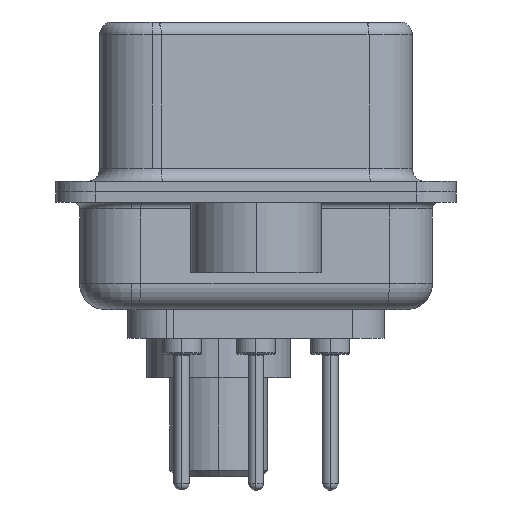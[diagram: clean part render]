
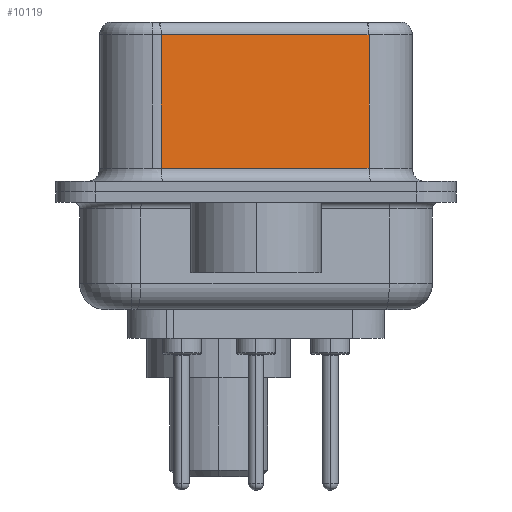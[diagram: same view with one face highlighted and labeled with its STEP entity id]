
A CAD part, left-side view. The second image highlights one B-rep face of the part: STEP entity #10119.
In plain terms, the highlighted planar face has unit normal (-0.985, -0.174, 0).
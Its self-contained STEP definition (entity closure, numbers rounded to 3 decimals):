
#584 = LINE ( 'NONE', #12378, #19956 ) ;
#1120 = CARTESIAN_POINT ( 'NONE',  ( 5.132, -4.322, 6.52 ) ) ;
#1971 = VECTOR ( 'NONE', #28779, 1000. ) ;
#3757 = VERTEX_POINT ( 'NONE', #9534 ) ;
#4213 = EDGE_LOOP ( 'NONE', ( #10689, #11433, #23676, #14604 ) ) ;
#5668 = DIRECTION ( 'NONE',  ( 0., 0., -1. ) ) ;
#5720 = PLANE ( 'NONE',  #8246 ) ;
#8246 = AXIS2_PLACEMENT_3D ( 'NONE', #1120, #19290, #12423 ) ;
#8667 = LINE ( 'NONE', #21960, #9747 ) ;
#9534 = CARTESIAN_POINT ( 'NONE',  ( 5.132, -4.322, 6.02 ) ) ;
#9747 = VECTOR ( 'NONE', #5668, 1000. ) ;
#9771 = VERTEX_POINT ( 'NONE', #20661 ) ;
#10119 = ADVANCED_FACE ( 'NONE', ( #22424 ), #5720, .F. ) ;
#10689 = ORIENTED_EDGE ( 'NONE', *, *, #27146, .F. ) ;
#11310 = VERTEX_POINT ( 'NONE', #18803 ) ;
#11433 = ORIENTED_EDGE ( 'NONE', *, *, #15634, .T. ) ;
#12378 = CARTESIAN_POINT ( 'NONE',  ( 5.132, -4.322, 0.9 ) ) ;
#12384 = LINE ( 'NONE', #28675, #1971 ) ;
#12423 = DIRECTION ( 'NONE',  ( -0.174, 0.985, 0. ) ) ;
#13137 = LINE ( 'NONE', #22871, #29001 ) ;
#14604 = ORIENTED_EDGE ( 'NONE', *, *, #19115, .T. ) ;
#15634 = EDGE_CURVE ( 'NONE', #3757, #27626, #13137, .T. ) ;
#18803 = CARTESIAN_POINT ( 'NONE',  ( 5.132, -4.322, 0.9 ) ) ;
#19115 = EDGE_CURVE ( 'NONE', #9771, #11310, #584, .T. ) ;
#19290 = DIRECTION ( 'NONE',  ( 0.985, 0.174, 0. ) ) ;
#19956 = VECTOR ( 'NONE', #25969, 1000. ) ;
#20661 = CARTESIAN_POINT ( 'NONE',  ( 3.73, 3.628, 0.9 ) ) ;
#21960 = CARTESIAN_POINT ( 'NONE',  ( 3.73, 3.628, 6.52 ) ) ;
#22424 = FACE_OUTER_BOUND ( 'NONE', #4213, .T. ) ;
#22871 = CARTESIAN_POINT ( 'NONE',  ( 5.132, -4.322, 6.02 ) ) ;
#23676 = ORIENTED_EDGE ( 'NONE', *, *, #29702, .T. ) ;
#25969 = DIRECTION ( 'NONE',  ( 0.174, -0.985, 0. ) ) ;
#27146 = EDGE_CURVE ( 'NONE', #3757, #11310, #12384, .T. ) ;
#27504 = DIRECTION ( 'NONE',  ( -0.174, 0.985, 0. ) ) ;
#27626 = VERTEX_POINT ( 'NONE', #28438 ) ;
#28438 = CARTESIAN_POINT ( 'NONE',  ( 3.73, 3.628, 6.02 ) ) ;
#28675 = CARTESIAN_POINT ( 'NONE',  ( 5.132, -4.322, 6.52 ) ) ;
#28779 = DIRECTION ( 'NONE',  ( 0., 0., -1. ) ) ;
#29001 = VECTOR ( 'NONE', #27504, 1000. ) ;
#29702 = EDGE_CURVE ( 'NONE', #27626, #9771, #8667, .T. ) ;
